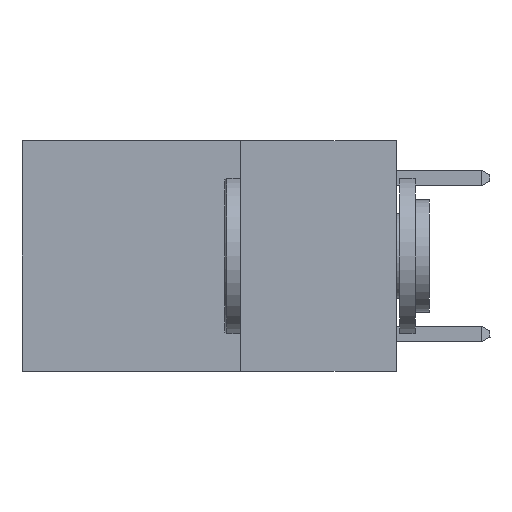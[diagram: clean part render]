
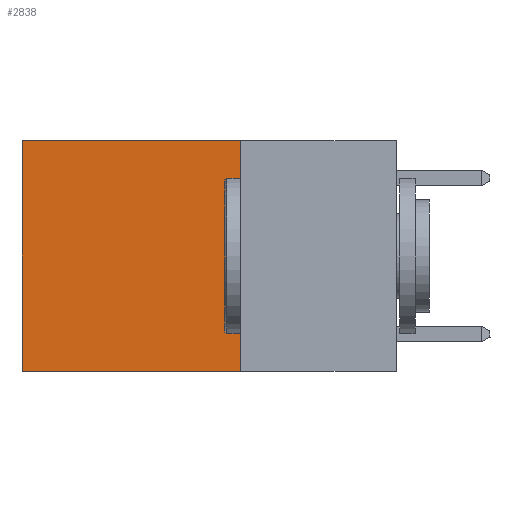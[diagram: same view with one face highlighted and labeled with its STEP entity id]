
A CAD part, left-side view. The second image highlights one B-rep face of the part: STEP entity #2838.
In plain terms, the highlighted planar face has unit normal (-1, 0, 0).
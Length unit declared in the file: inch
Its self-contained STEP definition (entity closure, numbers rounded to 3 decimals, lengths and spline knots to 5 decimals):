
#173 = ORIENTED_EDGE ( 'NONE', *, *, #12076, .F. ) ;
#196 = ORIENTED_EDGE ( 'NONE', *, *, #12681, .T. ) ;
#216 = PLANE ( 'NONE',  #5892 ) ;
#266 = CARTESIAN_POINT ( 'NONE',  ( 0.2625, 0.25, 0. ) ) ;
#588 = VERTEX_POINT ( 'NONE', #9361 ) ;
#594 = VECTOR ( 'NONE', #12049, 39.37008 ) ;
#1146 = EDGE_CURVE ( 'NONE', #3027, #8116, #8643, .T. ) ;
#1323 = VERTEX_POINT ( 'NONE', #12811 ) ;
#1495 = ORIENTED_EDGE ( 'NONE', *, *, #1146, .T. ) ;
#1930 = VECTOR ( 'NONE', #4171, 39.37008 ) ;
#2309 = DIRECTION ( 'NONE',  ( 0., 0., -1. ) ) ;
#2561 = DIRECTION ( 'NONE',  ( 0., 0., -1. ) ) ;
#2838 = ADVANCED_FACE ( 'NONE', ( #9042 ), #216, .F. ) ;
#2912 = CARTESIAN_POINT ( 'NONE',  ( 0.2625, 0.6, 0. ) ) ;
#3027 = VERTEX_POINT ( 'NONE', #9618 ) ;
#3268 = VECTOR ( 'NONE', #2561, 39.37008 ) ;
#3339 = EDGE_LOOP ( 'NONE', ( #1495, #8724, #173, #196 ) ) ;
#3841 = CARTESIAN_POINT ( 'NONE',  ( 0.2625, 0.6, -0.37 ) ) ;
#4171 = DIRECTION ( 'NONE',  ( 0., 0., -1. ) ) ;
#5405 = EDGE_CURVE ( 'NONE', #1323, #8116, #5976, .T. ) ;
#5686 = VECTOR ( 'NONE', #12395, 39.37008 ) ;
#5892 = AXIS2_PLACEMENT_3D ( 'NONE', #266, #8372, #2309 ) ;
#5976 = LINE ( 'NONE', #6998, #594 ) ;
#6023 = LINE ( 'NONE', #11386, #5686 ) ;
#6998 = CARTESIAN_POINT ( 'NONE',  ( 0.2625, 0.25, -0.37 ) ) ;
#7301 = LINE ( 'NONE', #8244, #1930 ) ;
#8116 = VERTEX_POINT ( 'NONE', #3841 ) ;
#8244 = CARTESIAN_POINT ( 'NONE',  ( 0.2625, 0.25, 0. ) ) ;
#8372 = DIRECTION ( 'NONE',  ( 1., 0., 0. ) ) ;
#8643 = LINE ( 'NONE', #2912, #3268 ) ;
#8724 = ORIENTED_EDGE ( 'NONE', *, *, #5405, .F. ) ;
#9042 = FACE_OUTER_BOUND ( 'NONE', #3339, .T. ) ;
#9361 = CARTESIAN_POINT ( 'NONE',  ( 0.2625, 0.25, 0. ) ) ;
#9618 = CARTESIAN_POINT ( 'NONE',  ( 0.2625, 0.6, 0. ) ) ;
#11386 = CARTESIAN_POINT ( 'NONE',  ( 0.2625, 0.25, 0. ) ) ;
#12049 = DIRECTION ( 'NONE',  ( 0., 1., 0. ) ) ;
#12076 = EDGE_CURVE ( 'NONE', #588, #1323, #7301, .T. ) ;
#12395 = DIRECTION ( 'NONE',  ( 0., 1., 0. ) ) ;
#12681 = EDGE_CURVE ( 'NONE', #588, #3027, #6023, .T. ) ;
#12811 = CARTESIAN_POINT ( 'NONE',  ( 0.2625, 0.25, -0.37 ) ) ;
